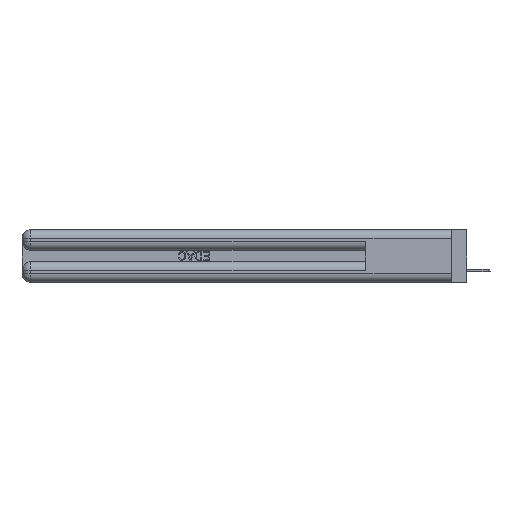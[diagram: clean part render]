
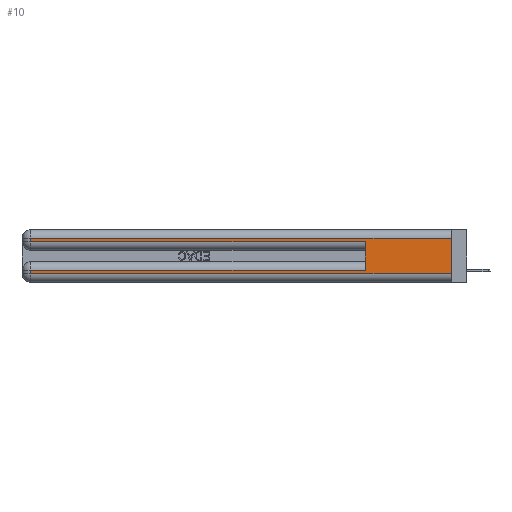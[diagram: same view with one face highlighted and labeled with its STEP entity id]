
A CAD part, left-side view. The second image highlights one B-rep face of the part: STEP entity #10.
In plain terms, the highlighted planar face has unit normal (-1, 0, 0).
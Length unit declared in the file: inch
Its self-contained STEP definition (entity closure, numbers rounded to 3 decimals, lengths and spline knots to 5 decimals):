
#10 = ADVANCED_FACE ( 'NONE', ( #29713 ), #51508, .F. ) ;
#400 = ORIENTED_EDGE ( 'NONE', *, *, #43080, .T. ) ;
#767 = VERTEX_POINT ( 'NONE', #23799 ) ;
#998 = VECTOR ( 'NONE', #43199, 39.37008 ) ;
#4049 = VERTEX_POINT ( 'NONE', #27134 ) ;
#4314 = CARTESIAN_POINT ( 'NONE',  ( 0., 0., 0.285 ) ) ;
#7340 = CARTESIAN_POINT ( 'NONE',  ( 0., 0.6, 0.145 ) ) ;
#7425 = LINE ( 'NONE', #51368, #998 ) ;
#7722 = VERTEX_POINT ( 'NONE', #41556 ) ;
#8676 = ORIENTED_EDGE ( 'NONE', *, *, #46679, .T. ) ;
#9537 = CARTESIAN_POINT ( 'NONE',  ( 0., 2.94, 0.085 ) ) ;
#10423 = CARTESIAN_POINT ( 'NONE',  ( 0., 0., 0.31 ) ) ;
#11791 = DIRECTION ( 'NONE',  ( 0., -1., 0. ) ) ;
#11941 = DIRECTION ( 'NONE',  ( 0., 0., -1. ) ) ;
#12604 = VERTEX_POINT ( 'NONE', #35957 ) ;
#13356 = CARTESIAN_POINT ( 'NONE',  ( 0., 2.94, 0.37 ) ) ;
#13910 = DIRECTION ( 'NONE',  ( 0., 1., 0. ) ) ;
#14083 = LINE ( 'NONE', #7340, #14757 ) ;
#14757 = VECTOR ( 'NONE', #32668, 39.37008 ) ;
#15507 = VECTOR ( 'NONE', #31236, 39.37008 ) ;
#16111 = ORIENTED_EDGE ( 'NONE', *, *, #39329, .T. ) ;
#17164 = DIRECTION ( 'NONE',  ( 0., -1., 0. ) ) ;
#18735 = ORIENTED_EDGE ( 'NONE', *, *, #50254, .T. ) ;
#20461 = CARTESIAN_POINT ( 'NONE',  ( 0., 0., 0.06 ) ) ;
#21519 = DIRECTION ( 'NONE',  ( 0., 0., -1. ) ) ;
#23660 = EDGE_CURVE ( 'NONE', #35137, #7722, #7425, .T. ) ;
#23799 = CARTESIAN_POINT ( 'NONE',  ( 0., 2.94, 0.06 ) ) ;
#24649 = ORIENTED_EDGE ( 'NONE', *, *, #27613, .T. ) ;
#24972 = VECTOR ( 'NONE', #21519, 39.37008 ) ;
#25072 = LINE ( 'NONE', #4314, #53686 ) ;
#27134 = CARTESIAN_POINT ( 'NONE',  ( 0., 2.94, 0.31 ) ) ;
#27255 = CARTESIAN_POINT ( 'NONE',  ( 0., 0., 0.37 ) ) ;
#27467 = CARTESIAN_POINT ( 'NONE',  ( 0., 0.6, 0.285 ) ) ;
#27613 = EDGE_CURVE ( 'NONE', #35137, #4049, #33622, .T. ) ;
#28209 = LINE ( 'NONE', #13356, #24972 ) ;
#28212 = ORIENTED_EDGE ( 'NONE', *, *, #36639, .T. ) ;
#29713 = FACE_OUTER_BOUND ( 'NONE', #41072, .T. ) ;
#30581 = VECTOR ( 'NONE', #11941, 39.37008 ) ;
#31052 = DIRECTION ( 'NONE',  ( 1., 0., 0. ) ) ;
#31236 = DIRECTION ( 'NONE',  ( 0., 1., 0. ) ) ;
#31257 = LINE ( 'NONE', #36695, #30581 ) ;
#32312 = LINE ( 'NONE', #20461, #44665 ) ;
#32668 = DIRECTION ( 'NONE',  ( 0., 0., 1. ) ) ;
#32717 = ORIENTED_EDGE ( 'NONE', *, *, #23660, .F. ) ;
#33622 = LINE ( 'NONE', #10423, #15507 ) ;
#35137 = VERTEX_POINT ( 'NONE', #40848 ) ;
#35835 = VECTOR ( 'NONE', #13910, 39.37008 ) ;
#35957 = CARTESIAN_POINT ( 'NONE',  ( 0., 0.6, 0.085 ) ) ;
#36639 = EDGE_CURVE ( 'NONE', #45280, #41333, #25072, .T. ) ;
#36695 = CARTESIAN_POINT ( 'NONE',  ( 0., 2.94, 0.37 ) ) ;
#38351 = CARTESIAN_POINT ( 'NONE',  ( 0., 0., 0.085 ) ) ;
#38610 = AXIS2_PLACEMENT_3D ( 'NONE', #27255, #31052, #47214 ) ;
#39329 = EDGE_CURVE ( 'NONE', #12604, #43447, #46904, .T. ) ;
#40848 = CARTESIAN_POINT ( 'NONE',  ( 0., 0., 0.31 ) ) ;
#41072 = EDGE_LOOP ( 'NONE', ( #32717, #24649, #400, #28212, #50984, #16111, #8676, #18735 ) ) ;
#41333 = VERTEX_POINT ( 'NONE', #27467 ) ;
#41556 = CARTESIAN_POINT ( 'NONE',  ( 0., 0., 0.06 ) ) ;
#43080 = EDGE_CURVE ( 'NONE', #4049, #45280, #31257, .T. ) ;
#43199 = DIRECTION ( 'NONE',  ( 0., 0., -1. ) ) ;
#43447 = VERTEX_POINT ( 'NONE', #9537 ) ;
#44665 = VECTOR ( 'NONE', #11791, 39.37008 ) ;
#45280 = VERTEX_POINT ( 'NONE', #45933 ) ;
#45933 = CARTESIAN_POINT ( 'NONE',  ( 0., 2.94, 0.285 ) ) ;
#46679 = EDGE_CURVE ( 'NONE', #43447, #767, #28209, .T. ) ;
#46904 = LINE ( 'NONE', #38351, #35835 ) ;
#47214 = DIRECTION ( 'NONE',  ( 0., 0., -1. ) ) ;
#50254 = EDGE_CURVE ( 'NONE', #767, #7722, #32312, .T. ) ;
#50961 = EDGE_CURVE ( 'NONE', #12604, #41333, #14083, .T. ) ;
#50984 = ORIENTED_EDGE ( 'NONE', *, *, #50961, .F. ) ;
#51368 = CARTESIAN_POINT ( 'NONE',  ( 0., 0., 0.37 ) ) ;
#51508 = PLANE ( 'NONE',  #38610 ) ;
#53686 = VECTOR ( 'NONE', #17164, 39.37008 ) ;
